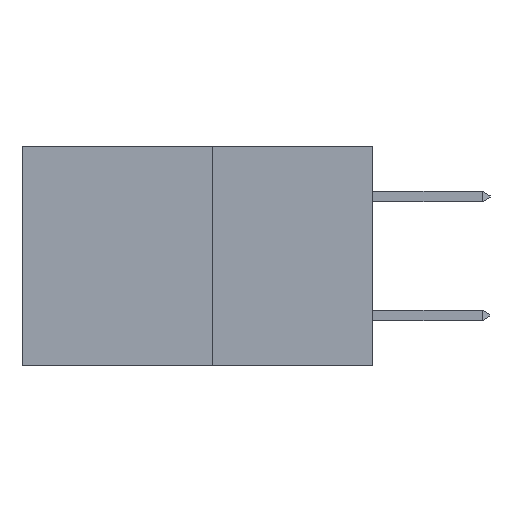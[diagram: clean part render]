
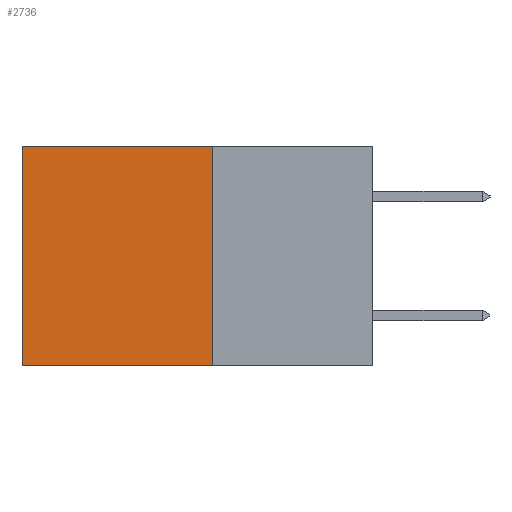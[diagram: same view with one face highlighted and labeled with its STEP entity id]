
A CAD part, left-side view. The second image highlights one B-rep face of the part: STEP entity #2736.
In plain terms, the highlighted planar face has unit normal (-1, 0, 0).
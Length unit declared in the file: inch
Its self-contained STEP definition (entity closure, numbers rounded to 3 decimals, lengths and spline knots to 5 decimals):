
#1698 = EDGE_CURVE ( 'NONE', #9103, #11949, #17551, .T. ) ;
#1861 = ORIENTED_EDGE ( 'NONE', *, *, #19834, .T. ) ;
#2736 = ADVANCED_FACE ( 'NONE', ( #13939 ), #7661, .F. ) ;
#6206 = DIRECTION ( 'NONE',  ( 0., 1., 0. ) ) ;
#6506 = DIRECTION ( 'NONE',  ( 0., 0., -1. ) ) ;
#6974 = DIRECTION ( 'NONE',  ( 0., 0., -1. ) ) ;
#7110 = CARTESIAN_POINT ( 'NONE',  ( 0.277, 0.59, -0.37 ) ) ;
#7149 = DIRECTION ( 'NONE',  ( 1., 0., 0. ) ) ;
#7243 = CARTESIAN_POINT ( 'NONE',  ( 0.277, 0.27, -0.37 ) ) ;
#7661 = PLANE ( 'NONE',  #15692 ) ;
#8200 = CARTESIAN_POINT ( 'NONE',  ( 0.277, 0.59, 0. ) ) ;
#8435 = LINE ( 'NONE', #18454, #16429 ) ;
#9103 = VERTEX_POINT ( 'NONE', #17592 ) ;
#9217 = VERTEX_POINT ( 'NONE', #8200 ) ;
#9504 = VECTOR ( 'NONE', #20335, 39.37008 ) ;
#10374 = EDGE_CURVE ( 'NONE', #11949, #19814, #21389, .T. ) ;
#11365 = EDGE_CURVE ( 'NONE', #9103, #9217, #18195, .T. ) ;
#11949 = VERTEX_POINT ( 'NONE', #16858 ) ;
#12695 = ORIENTED_EDGE ( 'NONE', *, *, #11365, .T. ) ;
#13921 = VECTOR ( 'NONE', #6206, 39.37008 ) ;
#13939 = FACE_OUTER_BOUND ( 'NONE', #19955, .T. ) ;
#14347 = ORIENTED_EDGE ( 'NONE', *, *, #10374, .F. ) ;
#15692 = AXIS2_PLACEMENT_3D ( 'NONE', #7243, #7149, #6974 ) ;
#16429 = VECTOR ( 'NONE', #20096, 39.37008 ) ;
#16858 = CARTESIAN_POINT ( 'NONE',  ( 0.277, 0.27, -0.37 ) ) ;
#17030 = VECTOR ( 'NONE', #6506, 39.37008 ) ;
#17454 = CARTESIAN_POINT ( 'NONE',  ( 0.277, 0.27, 0. ) ) ;
#17525 = ORIENTED_EDGE ( 'NONE', *, *, #1698, .F. ) ;
#17551 = LINE ( 'NONE', #18362, #17030 ) ;
#17592 = CARTESIAN_POINT ( 'NONE',  ( 0.277, 0.27, 0. ) ) ;
#18195 = LINE ( 'NONE', #17454, #13921 ) ;
#18362 = CARTESIAN_POINT ( 'NONE',  ( 0.277, 0.27, -0.37 ) ) ;
#18454 = CARTESIAN_POINT ( 'NONE',  ( 0.277, 0.59, -0.37 ) ) ;
#18667 = CARTESIAN_POINT ( 'NONE',  ( 0.277, 0.27, -0.37 ) ) ;
#19814 = VERTEX_POINT ( 'NONE', #7110 ) ;
#19834 = EDGE_CURVE ( 'NONE', #9217, #19814, #8435, .T. ) ;
#19955 = EDGE_LOOP ( 'NONE', ( #1861, #14347, #17525, #12695 ) ) ;
#20096 = DIRECTION ( 'NONE',  ( 0., 0., -1. ) ) ;
#20335 = DIRECTION ( 'NONE',  ( 0., 1., 0. ) ) ;
#21389 = LINE ( 'NONE', #18667, #9504 ) ;
